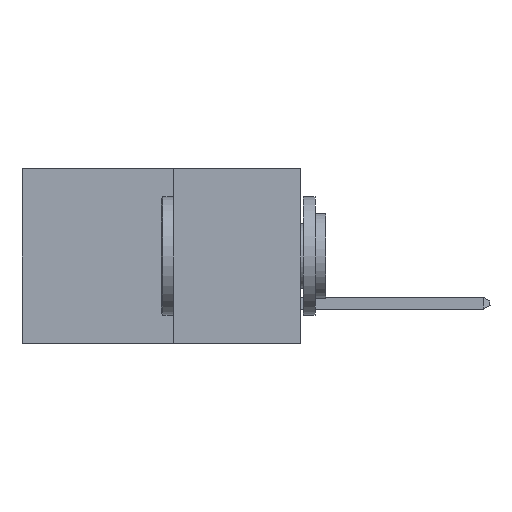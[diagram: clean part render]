
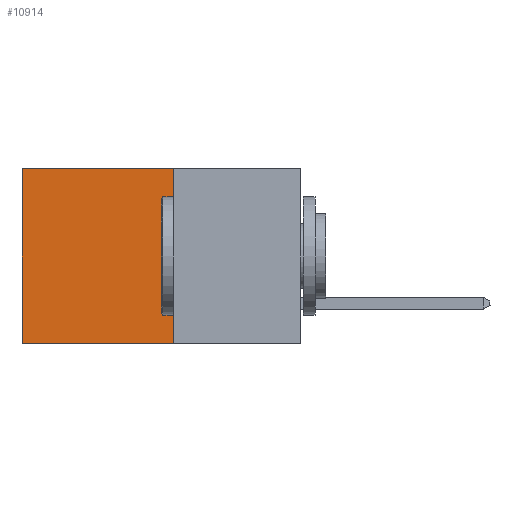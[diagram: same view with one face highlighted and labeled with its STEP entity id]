
A CAD part, left-side view. The second image highlights one B-rep face of the part: STEP entity #10914.
In plain terms, the highlighted planar face has unit normal (-1, 0, 0).
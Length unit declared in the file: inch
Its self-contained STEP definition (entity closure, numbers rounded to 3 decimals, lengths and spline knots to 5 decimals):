
#335 = CARTESIAN_POINT ( 'NONE',  ( 0.277, 0.27, -0.37 ) ) ;
#627 = DIRECTION ( 'NONE',  ( 0., 0., -1. ) ) ;
#663 = CARTESIAN_POINT ( 'NONE',  ( 0.277, 0.59, -0.37 ) ) ;
#1297 = DIRECTION ( 'NONE',  ( 0., 1., 0. ) ) ;
#1373 = CARTESIAN_POINT ( 'NONE',  ( 0.277, 0.27, -0.37 ) ) ;
#1714 = DIRECTION ( 'NONE',  ( 1., 0., 0. ) ) ;
#1941 = DIRECTION ( 'NONE',  ( 0., 0., -1. ) ) ;
#3259 = CARTESIAN_POINT ( 'NONE',  ( 0.277, 0.27, -0.37 ) ) ;
#4236 = EDGE_CURVE ( 'NONE', #15766, #9368, #19362, .T. ) ;
#4378 = VECTOR ( 'NONE', #6738, 39.37008 ) ;
#4783 = CARTESIAN_POINT ( 'NONE',  ( 0.277, 0.59, 0. ) ) ;
#6377 = ORIENTED_EDGE ( 'NONE', *, *, #19701, .T. ) ;
#6738 = DIRECTION ( 'NONE',  ( 0., 1., 0. ) ) ;
#7101 = ORIENTED_EDGE ( 'NONE', *, *, #4236, .F. ) ;
#7108 = EDGE_CURVE ( 'NONE', #10853, #9368, #12738, .T. ) ;
#8689 = CARTESIAN_POINT ( 'NONE',  ( 0.277, 0.59, -0.37 ) ) ;
#9368 = VERTEX_POINT ( 'NONE', #8689 ) ;
#9765 = LINE ( 'NONE', #335, #17290 ) ;
#10680 = AXIS2_PLACEMENT_3D ( 'NONE', #3259, #1714, #12696 ) ;
#10853 = VERTEX_POINT ( 'NONE', #4783 ) ;
#10860 = FACE_OUTER_BOUND ( 'NONE', #17576, .T. ) ;
#10914 = ADVANCED_FACE ( 'NONE', ( #10860 ), #11200, .F. ) ;
#11200 = PLANE ( 'NONE',  #10680 ) ;
#12696 = DIRECTION ( 'NONE',  ( 0., 0., -1. ) ) ;
#12738 = LINE ( 'NONE', #663, #16242 ) ;
#13331 = CARTESIAN_POINT ( 'NONE',  ( 0.277, 0.27, 0. ) ) ;
#15766 = VERTEX_POINT ( 'NONE', #18036 ) ;
#15843 = VECTOR ( 'NONE', #1297, 39.37008 ) ;
#15901 = CARTESIAN_POINT ( 'NONE',  ( 0.277, 0.27, 0. ) ) ;
#16242 = VECTOR ( 'NONE', #627, 39.37008 ) ;
#16335 = EDGE_CURVE ( 'NONE', #18499, #15766, #9765, .T. ) ;
#16700 = ORIENTED_EDGE ( 'NONE', *, *, #16335, .F. ) ;
#17290 = VECTOR ( 'NONE', #1941, 39.37008 ) ;
#17576 = EDGE_LOOP ( 'NONE', ( #18949, #7101, #16700, #6377 ) ) ;
#18036 = CARTESIAN_POINT ( 'NONE',  ( 0.277, 0.27, -0.37 ) ) ;
#18499 = VERTEX_POINT ( 'NONE', #13331 ) ;
#18949 = ORIENTED_EDGE ( 'NONE', *, *, #7108, .T. ) ;
#19362 = LINE ( 'NONE', #1373, #15843 ) ;
#19693 = LINE ( 'NONE', #15901, #4378 ) ;
#19701 = EDGE_CURVE ( 'NONE', #18499, #10853, #19693, .T. ) ;
